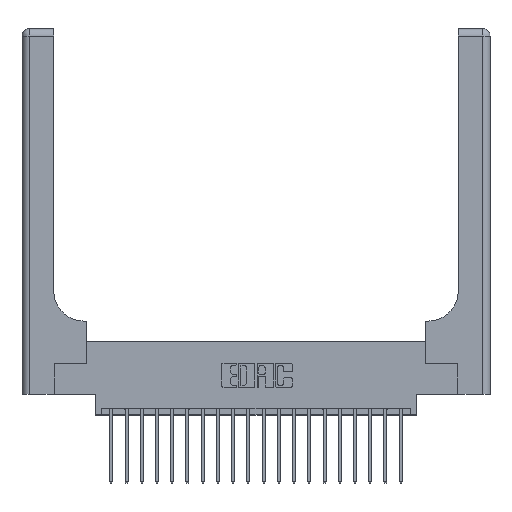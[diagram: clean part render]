
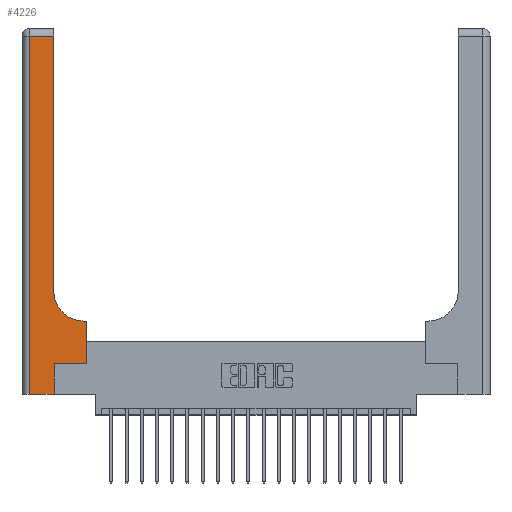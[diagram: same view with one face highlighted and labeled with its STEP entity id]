
A CAD part, top view. The second image highlights one B-rep face of the part: STEP entity #4226.
In plain terms, the highlighted planar face has unit normal (0, 0, 1).
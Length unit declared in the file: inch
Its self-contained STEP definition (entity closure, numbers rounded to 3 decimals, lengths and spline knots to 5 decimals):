
#39 = CARTESIAN_POINT ( 'NONE',  ( 0.528, 0.25, 0.37 ) ) ;
#547 = ORIENTED_EDGE ( 'NONE', *, *, #5151, .T. ) ;
#719 = LINE ( 'NONE', #13846, #15478 ) ;
#1033 = VERTEX_POINT ( 'NONE', #13789 ) ;
#1482 = CARTESIAN_POINT ( 'NONE',  ( 0.26, 3., 0.37 ) ) ;
#1704 = LINE ( 'NONE', #1482, #11467 ) ;
#2959 = DIRECTION ( 'NONE',  ( 0., 1., 0. ) ) ;
#3532 = AXIS2_PLACEMENT_3D ( 'NONE', #4660, #21554, #4987 ) ;
#3573 = VERTEX_POINT ( 'NONE', #3601 ) ;
#3601 = CARTESIAN_POINT ( 'NONE',  ( 0.265, 0.25, 0.37 ) ) ;
#3609 = DIRECTION ( 'NONE',  ( 0., -1., 0. ) ) ;
#3618 = DIRECTION ( 'NONE',  ( -1., 0., 0. ) ) ;
#3699 = VECTOR ( 'NONE', #3609, 39.37008 ) ;
#4099 = VECTOR ( 'NONE', #18232, 39.37008 ) ;
#4226 = ADVANCED_FACE ( 'NONE', ( #9608 ), #8063, .F. ) ;
#4259 = ORIENTED_EDGE ( 'NONE', *, *, #19511, .T. ) ;
#4660 = CARTESIAN_POINT ( 'NONE',  ( 0.51, 0.85, 0.37 ) ) ;
#4770 = CARTESIAN_POINT ( 'NONE',  ( 0.265, 0.25, 0.37 ) ) ;
#4987 = DIRECTION ( 'NONE',  ( 1., 0., 0. ) ) ;
#5151 = EDGE_CURVE ( 'NONE', #1033, #9020, #19650, .T. ) ;
#5256 = CIRCLE ( 'NONE', #3532, 0.25 ) ;
#5349 = CARTESIAN_POINT ( 'NONE',  ( 0., 0., 0.37 ) ) ;
#5438 = VERTEX_POINT ( 'NONE', #14778 ) ;
#6025 = LINE ( 'NONE', #12752, #14392 ) ;
#6100 = LINE ( 'NONE', #17804, #6978 ) ;
#6160 = CARTESIAN_POINT ( 'NONE',  ( 0.265, 0., 0.37 ) ) ;
#6257 = VERTEX_POINT ( 'NONE', #12858 ) ;
#6978 = VECTOR ( 'NONE', #21007, 39.37008 ) ;
#7421 = ORIENTED_EDGE ( 'NONE', *, *, #21596, .T. ) ;
#8063 = PLANE ( 'NONE',  #11018 ) ;
#8195 = DIRECTION ( 'NONE',  ( 0., 1., 0. ) ) ;
#8459 = CARTESIAN_POINT ( 'NONE',  ( 0.06, 3., 0.37 ) ) ;
#8587 = ORIENTED_EDGE ( 'NONE', *, *, #13794, .T. ) ;
#8673 = DIRECTION ( 'NONE',  ( 1., 0., 0. ) ) ;
#9020 = VERTEX_POINT ( 'NONE', #19258 ) ;
#9239 = ORIENTED_EDGE ( 'NONE', *, *, #13815, .T. ) ;
#9519 = EDGE_CURVE ( 'NONE', #6257, #20652, #719, .T. ) ;
#9608 = FACE_OUTER_BOUND ( 'NONE', #15138, .T. ) ;
#9622 = EDGE_CURVE ( 'NONE', #9020, #5438, #6100, .T. ) ;
#9894 = VERTEX_POINT ( 'NONE', #13824 ) ;
#10106 = ORIENTED_EDGE ( 'NONE', *, *, #9622, .T. ) ;
#10928 = CARTESIAN_POINT ( 'NONE',  ( 0.26, 0.85, 0.37 ) ) ;
#11018 = AXIS2_PLACEMENT_3D ( 'NONE', #14772, #21535, #16321 ) ;
#11086 = VECTOR ( 'NONE', #8673, 39.37008 ) ;
#11467 = VECTOR ( 'NONE', #8195, 39.37008 ) ;
#11521 = LINE ( 'NONE', #4770, #13009 ) ;
#11984 = LINE ( 'NONE', #5349, #11086 ) ;
#12351 = CARTESIAN_POINT ( 'NONE',  ( 0.06, 2.94, 0.37 ) ) ;
#12752 = CARTESIAN_POINT ( 'NONE',  ( 0.265, 0., 0.37 ) ) ;
#12858 = CARTESIAN_POINT ( 'NONE',  ( 0.26, 2.94, 0.37 ) ) ;
#12996 = EDGE_CURVE ( 'NONE', #20332, #6257, #1704, .T. ) ;
#13009 = VECTOR ( 'NONE', #16572, 39.37008 ) ;
#13789 = CARTESIAN_POINT ( 'NONE',  ( 0.528, 0.25, 0.37 ) ) ;
#13794 = EDGE_CURVE ( 'NONE', #9894, #17710, #11984, .T. ) ;
#13815 = EDGE_CURVE ( 'NONE', #20652, #9894, #18701, .T. ) ;
#13824 = CARTESIAN_POINT ( 'NONE',  ( 0.06, 0., 0.37 ) ) ;
#13846 = CARTESIAN_POINT ( 'NONE',  ( 0., 2.94, 0.37 ) ) ;
#14392 = VECTOR ( 'NONE', #2959, 39.37008 ) ;
#14772 = CARTESIAN_POINT ( 'NONE',  ( 0., 3., 0.37 ) ) ;
#14778 = CARTESIAN_POINT ( 'NONE',  ( 0.51, 0.6, 0.37 ) ) ;
#14951 = ORIENTED_EDGE ( 'NONE', *, *, #12996, .T. ) ;
#15138 = EDGE_LOOP ( 'NONE', ( #14951, #16661, #9239, #8587, #4259, #19592, #547, #10106, #7421 ) ) ;
#15478 = VECTOR ( 'NONE', #3618, 39.37008 ) ;
#16321 = DIRECTION ( 'NONE',  ( -1., 0., 0. ) ) ;
#16572 = DIRECTION ( 'NONE',  ( 1., 0., 0. ) ) ;
#16661 = ORIENTED_EDGE ( 'NONE', *, *, #9519, .T. ) ;
#17710 = VERTEX_POINT ( 'NONE', #6160 ) ;
#17804 = CARTESIAN_POINT ( 'NONE',  ( 0.26, 0.6, 0.37 ) ) ;
#18232 = DIRECTION ( 'NONE',  ( 0., 1., 0. ) ) ;
#18701 = LINE ( 'NONE', #8459, #3699 ) ;
#19258 = CARTESIAN_POINT ( 'NONE',  ( 0.528, 0.6, 0.37 ) ) ;
#19511 = EDGE_CURVE ( 'NONE', #17710, #3573, #6025, .T. ) ;
#19592 = ORIENTED_EDGE ( 'NONE', *, *, #21581, .T. ) ;
#19650 = LINE ( 'NONE', #39, #4099 ) ;
#20332 = VERTEX_POINT ( 'NONE', #10928 ) ;
#20652 = VERTEX_POINT ( 'NONE', #12351 ) ;
#21007 = DIRECTION ( 'NONE',  ( -1., 0., 0. ) ) ;
#21535 = DIRECTION ( 'NONE',  ( 0., 0., -1. ) ) ;
#21554 = DIRECTION ( 'NONE',  ( 0., 0., -1. ) ) ;
#21581 = EDGE_CURVE ( 'NONE', #3573, #1033, #11521, .T. ) ;
#21596 = EDGE_CURVE ( 'NONE', #5438, #20332, #5256, .T. ) ;
